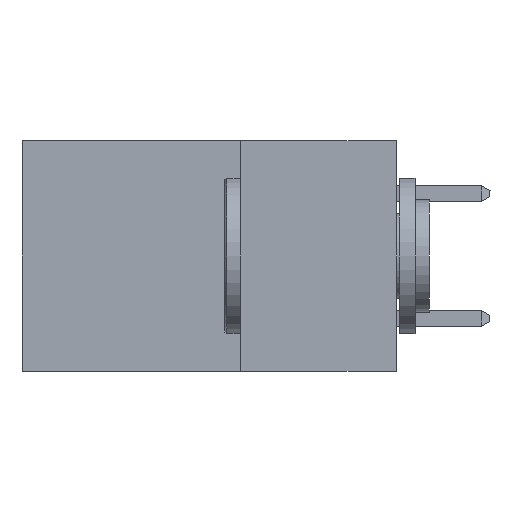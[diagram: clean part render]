
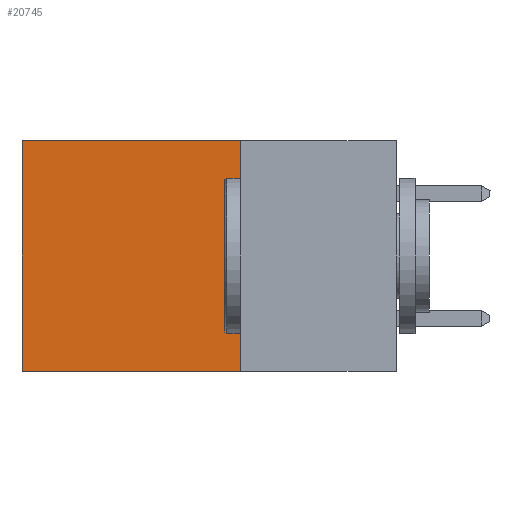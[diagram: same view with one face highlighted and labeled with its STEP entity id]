
A CAD part, left-side view. The second image highlights one B-rep face of the part: STEP entity #20745.
In plain terms, the highlighted planar face has unit normal (-1, 0, 0).
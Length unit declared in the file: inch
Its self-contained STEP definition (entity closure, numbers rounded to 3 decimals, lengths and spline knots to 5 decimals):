
#68 = EDGE_CURVE ( 'NONE', #1724, #16573, #13406, .T. ) ;
#390 = VERTEX_POINT ( 'NONE', #13809 ) ;
#1660 = ORIENTED_EDGE ( 'NONE', *, *, #2377, .F. ) ;
#1724 = VERTEX_POINT ( 'NONE', #18750 ) ;
#2377 = EDGE_CURVE ( 'NONE', #390, #14710, #20029, .T. ) ;
#2501 = VECTOR ( 'NONE', #17103, 39.37008 ) ;
#3199 = DIRECTION ( 'NONE',  ( 0., 0., -1. ) ) ;
#3728 = CARTESIAN_POINT ( 'NONE',  ( 0.298, 0.6, -0.37 ) ) ;
#4360 = DIRECTION ( 'NONE',  ( 0., 1., 0. ) ) ;
#4678 = ORIENTED_EDGE ( 'NONE', *, *, #22225, .F. ) ;
#5233 = LINE ( 'NONE', #8497, #2501 ) ;
#8497 = CARTESIAN_POINT ( 'NONE',  ( 0.298, 0.25, -0.37 ) ) ;
#8872 = DIRECTION ( 'NONE',  ( 0., 0., -1. ) ) ;
#9948 = ORIENTED_EDGE ( 'NONE', *, *, #16659, .T. ) ;
#10707 = VECTOR ( 'NONE', #8872, 39.37008 ) ;
#12488 = CARTESIAN_POINT ( 'NONE',  ( 0.298, 0.6, 0. ) ) ;
#13342 = PLANE ( 'NONE',  #22210 ) ;
#13406 = LINE ( 'NONE', #12488, #10707 ) ;
#13570 = FACE_OUTER_BOUND ( 'NONE', #21558, .T. ) ;
#13809 = CARTESIAN_POINT ( 'NONE',  ( 0.298, 0.25, 0. ) ) ;
#14117 = VECTOR ( 'NONE', #17679, 39.37008 ) ;
#14633 = CARTESIAN_POINT ( 'NONE',  ( 0.298, 0.25, 0. ) ) ;
#14710 = VERTEX_POINT ( 'NONE', #16747 ) ;
#15382 = DIRECTION ( 'NONE',  ( 1., 0., 0. ) ) ;
#16573 = VERTEX_POINT ( 'NONE', #3728 ) ;
#16659 = EDGE_CURVE ( 'NONE', #390, #1724, #21269, .T. ) ;
#16747 = CARTESIAN_POINT ( 'NONE',  ( 0.298, 0.25, -0.37 ) ) ;
#17103 = DIRECTION ( 'NONE',  ( 0., 1., 0. ) ) ;
#17679 = DIRECTION ( 'NONE',  ( 0., 0., -1. ) ) ;
#18551 = VECTOR ( 'NONE', #4360, 39.37008 ) ;
#18750 = CARTESIAN_POINT ( 'NONE',  ( 0.298, 0.6, 0. ) ) ;
#20019 = ORIENTED_EDGE ( 'NONE', *, *, #68, .T. ) ;
#20029 = LINE ( 'NONE', #21162, #14117 ) ;
#20745 = ADVANCED_FACE ( 'NONE', ( #13570 ), #13342, .F. ) ;
#21162 = CARTESIAN_POINT ( 'NONE',  ( 0.298, 0.25, 0. ) ) ;
#21269 = LINE ( 'NONE', #14633, #18551 ) ;
#21558 = EDGE_LOOP ( 'NONE', ( #20019, #4678, #1660, #9948 ) ) ;
#22210 = AXIS2_PLACEMENT_3D ( 'NONE', #22227, #15382, #3199 ) ;
#22225 = EDGE_CURVE ( 'NONE', #14710, #16573, #5233, .T. ) ;
#22227 = CARTESIAN_POINT ( 'NONE',  ( 0.298, 0.25, 0. ) ) ;
